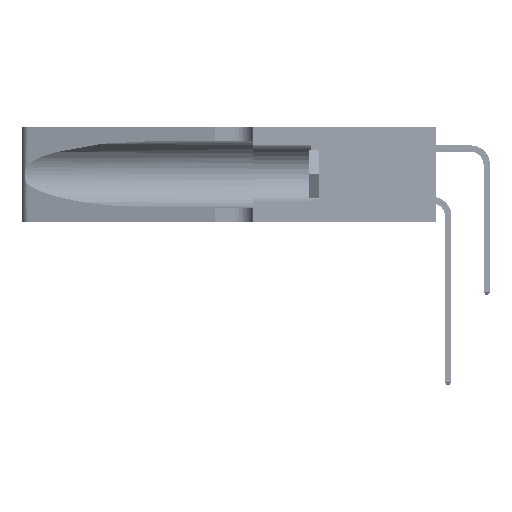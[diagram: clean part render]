
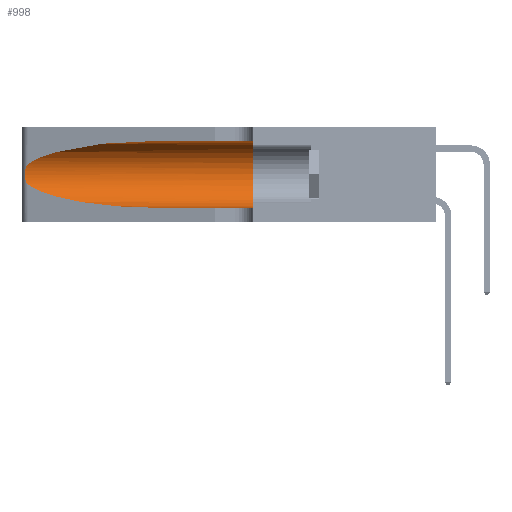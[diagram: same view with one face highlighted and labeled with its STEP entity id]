
A CAD part, left-side view. The second image highlights one B-rep face of the part: STEP entity #998.
In plain terms, the highlighted cylindrical face has radius 3.308 mm (diameter 6.617 mm), a partial arc.
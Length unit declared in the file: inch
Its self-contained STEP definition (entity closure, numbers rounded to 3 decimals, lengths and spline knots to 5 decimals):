
#998 = ADVANCED_FACE ( 'NONE', ( #45353 ), #11216, .F. ) ;
#1728 = EDGE_CURVE ( 'NONE', #15173, #17459, #35882, .T. ) ;
#3209 = CARTESIAN_POINT ( 'NONE',  ( 0.26075, 1.23896, 0.19203 ) ) ;
#3916 = VERTEX_POINT ( 'NONE', #47875 ) ;
#4342 = CARTESIAN_POINT ( 'NONE',  ( 0.2373, 1.15595, 0.08982 ) ) ;
#4516 = EDGE_CURVE ( 'NONE', #40942, #15173, #5972, .T. ) ;
#4907 = CARTESIAN_POINT ( 'NONE',  ( 0.1305, 0.35, 0.05475 ) ) ;
#5799 = CARTESIAN_POINT ( 'NONE',  ( 0.25487, 1.22718, 0.22369 ) ) ;
#5849 = CARTESIAN_POINT ( 'NONE',  ( 0.18966, 0.96281, 0.31525 ) ) ;
#5972 = B_SPLINE_CURVE_WITH_KNOTS ( 'NONE', 3,
 ( #18923, #35709, #39781, #31706, #30956, #24221, #3209, #48530, #37309, #48373, #6662, #44669, #10744, #7137 ),
 .UNSPECIFIED., .F., .F.,
 ( 4, 2, 2, 2, 2, 2, 4 ),
 ( 0., 0.00027, 0.00053, 0.00107, 0.0016, 0.00187, 0.00214 ),
 .UNSPECIFIED. ) ;
#6208 = CARTESIAN_POINT ( 'NONE',  ( 0.25487, 1.22718, 0.14631 ) ) ;
#6662 = CARTESIAN_POINT ( 'NONE',  ( 0.25789, 1.23486, 0.15765 ) ) ;
#7137 = CARTESIAN_POINT ( 'NONE',  ( 0.25487, 1.22718, 0.14631 ) ) ;
#7191 = CARTESIAN_POINT ( 'NONE',  ( 0.1305, 0.72297, 0.05475 ) ) ;
#7365 = LINE ( 'NONE', #26920, #36283 ) ;
#8589 = VERTEX_POINT ( 'NONE', #9035 ) ;
#8826 = DIRECTION ( 'NONE',  ( 0., -1., 0. ) ) ;
#9035 = CARTESIAN_POINT ( 'NONE',  ( 0.1305, 0.72297, 0.31525 ) ) ;
#9158 = DIRECTION ( 'NONE',  ( 0., 0., -1. ) ) ;
#9187 = LINE ( 'NONE', #31403, #17454 ) ;
#9734 = AXIS2_PLACEMENT_3D ( 'NONE', #17047, #8826, #9158 ) ;
#10744 = CARTESIAN_POINT ( 'NONE',  ( 0.25555, 1.22993, 0.14849 ) ) ;
#11216 = CYLINDRICAL_SURFACE ( 'NONE', #9734, 0.13025 ) ;
#14998 = EDGE_CURVE ( 'NONE', #17459, #21833, #9187, .T. ) ;
#15173 = VERTEX_POINT ( 'NONE', #6208 ) ;
#17011 = CARTESIAN_POINT ( 'NONE',  ( 0.2373, 1.15595, 0.28018 ) ) ;
#17047 = CARTESIAN_POINT ( 'NONE',  ( 0.1305, 1.61858, 0.185 ) ) ;
#17181 = EDGE_LOOP ( 'NONE', ( #22058, #42574, #29062, #34338, #38989, #45156 ) ) ;
#17454 = VECTOR ( 'NONE', #35371, 39.37008 ) ;
#17459 = VERTEX_POINT ( 'NONE', #7191 ) ;
#18923 = CARTESIAN_POINT ( 'NONE',  ( 0.25487, 1.22718, 0.22369 ) ) ;
#19980 = AXIS2_PLACEMENT_3D ( 'NONE', #26880, #26391, #26547 ) ;
#20830 = CARTESIAN_POINT ( 'NONE',  ( 0.25487, 1.22718, 0.22369 ) ) ;
#21146 = CARTESIAN_POINT ( 'NONE',  ( 0.1305, 0.72297, 0.31525 ) ) ;
#21833 = VERTEX_POINT ( 'NONE', #4907 ) ;
#22058 = ORIENTED_EDGE ( 'NONE', *, *, #40399, .T. ) ;
#23129 = DIRECTION ( 'NONE',  ( 0., -1., 0. ) ) ;
#23425 = CARTESIAN_POINT ( 'NONE',  ( 0.1305, 0.72297, 0.05475 ) ) ;
#24221 = CARTESIAN_POINT ( 'NONE',  ( 0.26018, 1.23835, 0.19895 ) ) ;
#26391 = DIRECTION ( 'NONE',  ( 0., 1., 0. ) ) ;
#26547 = DIRECTION ( 'NONE',  ( 0., 0., 1. ) ) ;
#26880 = CARTESIAN_POINT ( 'NONE',  ( 0.1305, 0.35, 0.185 ) ) ;
#26920 = CARTESIAN_POINT ( 'NONE',  ( 0.1305, 1.61858, 0.31525 ) ) ;
#29062 = ORIENTED_EDGE ( 'NONE', *, *, #1728, .T. ) ;
#29467 = EDGE_CURVE ( 'NONE', #3916, #21833, #43224, .T. ) ;
#30666 = CARTESIAN_POINT ( 'NONE',  ( 0.18966, 0.96281, 0.05475 ) ) ;
#30956 = CARTESIAN_POINT ( 'NONE',  ( 0.25854, 1.2359, 0.20912 ) ) ;
#31403 = CARTESIAN_POINT ( 'NONE',  ( 0.1305, 1.61858, 0.05475 ) ) ;
#31706 = CARTESIAN_POINT ( 'NONE',  ( 0.25787, 1.23484, 0.2124 ) ) ;
#34338 = ORIENTED_EDGE ( 'NONE', *, *, #14998, .T. ) ;
#34981 =( BOUNDED_CURVE ( )  B_SPLINE_CURVE ( 3, ( #21146, #5849, #17011, #20830 ),
 .UNSPECIFIED., .F., .F. ) 
 B_SPLINE_CURVE_WITH_KNOTS ( ( 4, 4 ),
 ( 1.5708, 2.84003 ),
 .UNSPECIFIED. ) 
 CURVE ( )  GEOMETRIC_REPRESENTATION_ITEM ( )  RATIONAL_B_SPLINE_CURVE ( ( 1., 0.87, 0.87, 1. ) ) 
 REPRESENTATION_ITEM ( '' )  );
#35371 = DIRECTION ( 'NONE',  ( 0., -1., 0. ) ) ;
#35709 = CARTESIAN_POINT ( 'NONE',  ( 0.25555, 1.22994, 0.2215 ) ) ;
#35882 =( BOUNDED_CURVE ( )  B_SPLINE_CURVE ( 3, ( #38299, #4342, #30666, #23425 ),
 .UNSPECIFIED., .F., .F. ) 
 B_SPLINE_CURVE_WITH_KNOTS ( ( 4, 4 ),
 ( 3.44316, 4.71239 ),
 .UNSPECIFIED. ) 
 CURVE ( )  GEOMETRIC_REPRESENTATION_ITEM ( )  RATIONAL_B_SPLINE_CURVE ( ( 1., 0.87, 0.87, 1. ) ) 
 REPRESENTATION_ITEM ( '' )  );
#36283 = VECTOR ( 'NONE', #23129, 39.37008 ) ;
#37309 = CARTESIAN_POINT ( 'NONE',  ( 0.26017, 1.23833, 0.17102 ) ) ;
#38299 = CARTESIAN_POINT ( 'NONE',  ( 0.25487, 1.22718, 0.14631 ) ) ;
#38989 = ORIENTED_EDGE ( 'NONE', *, *, #29467, .F. ) ;
#39781 = CARTESIAN_POINT ( 'NONE',  ( 0.25639, 1.23184, 0.21858 ) ) ;
#40025 = EDGE_CURVE ( 'NONE', #8589, #3916, #7365, .T. ) ;
#40399 = EDGE_CURVE ( 'NONE', #8589, #40942, #34981, .T. ) ;
#40942 = VERTEX_POINT ( 'NONE', #5799 ) ;
#42574 = ORIENTED_EDGE ( 'NONE', *, *, #4516, .T. ) ;
#43224 = CIRCLE ( 'NONE', #19980, 0.13025 ) ;
#44669 = CARTESIAN_POINT ( 'NONE',  ( 0.25639, 1.23186, 0.15144 ) ) ;
#45156 = ORIENTED_EDGE ( 'NONE', *, *, #40025, .F. ) ;
#45353 = FACE_OUTER_BOUND ( 'NONE', #17181, .T. ) ;
#47875 = CARTESIAN_POINT ( 'NONE',  ( 0.1305, 0.35, 0.31525 ) ) ;
#48373 = CARTESIAN_POINT ( 'NONE',  ( 0.25856, 1.23593, 0.16098 ) ) ;
#48530 = CARTESIAN_POINT ( 'NONE',  ( 0.26075, 1.23896, 0.178 ) ) ;
